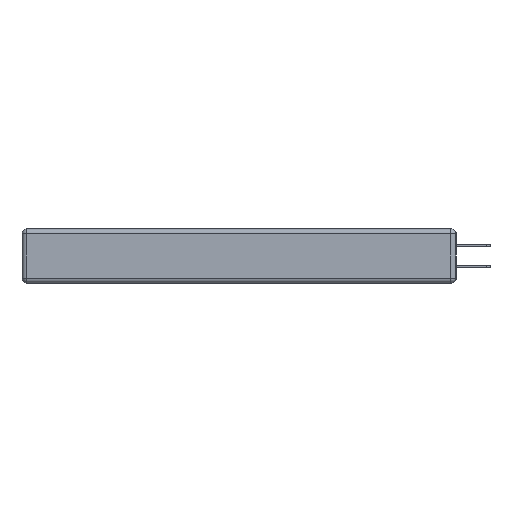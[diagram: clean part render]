
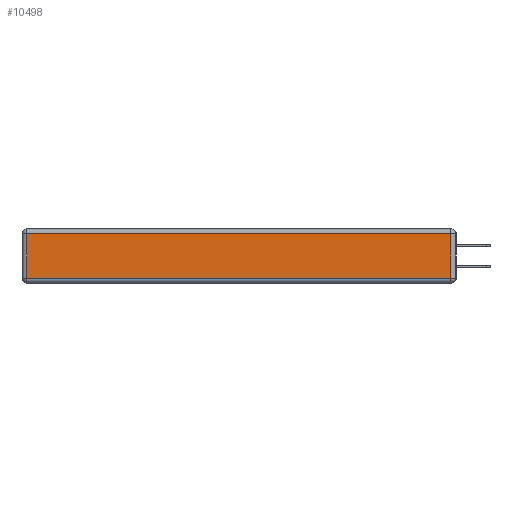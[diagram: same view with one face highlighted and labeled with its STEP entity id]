
A CAD part, left-side view. The second image highlights one B-rep face of the part: STEP entity #10498.
In plain terms, the highlighted planar face has unit normal (-1, 0, 0).
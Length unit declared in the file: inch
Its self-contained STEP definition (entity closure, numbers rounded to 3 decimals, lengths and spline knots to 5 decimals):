
#58 = CARTESIAN_POINT ( 'NONE',  ( 0., 0., -0.313 ) ) ;
#170 = CARTESIAN_POINT ( 'NONE',  ( 0., 0.03, -0.313 ) ) ;
#634 = ORIENTED_EDGE ( 'NONE', *, *, #1291, .T. ) ;
#694 = VECTOR ( 'NONE', #5084, 39.37008 ) ;
#899 = EDGE_CURVE ( 'NONE', #4016, #5563, #7367, .T. ) ;
#963 = VERTEX_POINT ( 'NONE', #13430 ) ;
#1291 = EDGE_CURVE ( 'NONE', #5563, #10634, #12744, .T. ) ;
#1335 = DIRECTION ( 'NONE',  ( 0., 0., 1. ) ) ;
#1717 = EDGE_LOOP ( 'NONE', ( #12720, #4150, #634, #4134 ) ) ;
#2519 = DIRECTION ( 'NONE',  ( -1., 0., 0. ) ) ;
#2928 = LINE ( 'NONE', #58, #13355 ) ;
#2948 = EDGE_CURVE ( 'NONE', #963, #4016, #2928, .T. ) ;
#3282 = DIRECTION ( 'NONE',  ( 0., -1., 0. ) ) ;
#3499 = CARTESIAN_POINT ( 'NONE',  ( 0., 2.75, -0.03 ) ) ;
#4013 = LINE ( 'NONE', #4587, #4160 ) ;
#4016 = VERTEX_POINT ( 'NONE', #170 ) ;
#4134 = ORIENTED_EDGE ( 'NONE', *, *, #13075, .T. ) ;
#4150 = ORIENTED_EDGE ( 'NONE', *, *, #899, .T. ) ;
#4160 = VECTOR ( 'NONE', #12890, 39.37008 ) ;
#4257 = AXIS2_PLACEMENT_3D ( 'NONE', #8532, #2519, #1335 ) ;
#4587 = CARTESIAN_POINT ( 'NONE',  ( 0., 2.72, -0.343 ) ) ;
#5084 = DIRECTION ( 'NONE',  ( 0., 0., 1. ) ) ;
#5414 = VECTOR ( 'NONE', #11889, 39.37008 ) ;
#5563 = VERTEX_POINT ( 'NONE', #9408 ) ;
#6183 = CARTESIAN_POINT ( 'NONE',  ( 0., 2.72, -0.03 ) ) ;
#7300 = CARTESIAN_POINT ( 'NONE',  ( 0., 0.03, -0.343 ) ) ;
#7367 = LINE ( 'NONE', #7300, #694 ) ;
#8532 = CARTESIAN_POINT ( 'NONE',  ( 0., 0., -0.343 ) ) ;
#9408 = CARTESIAN_POINT ( 'NONE',  ( 0., 0.03, -0.03 ) ) ;
#10498 = ADVANCED_FACE ( 'NONE', ( #11075 ), #11639, .T. ) ;
#10634 = VERTEX_POINT ( 'NONE', #6183 ) ;
#11075 = FACE_OUTER_BOUND ( 'NONE', #1717, .T. ) ;
#11639 = PLANE ( 'NONE',  #4257 ) ;
#11889 = DIRECTION ( 'NONE',  ( 0., 1., 0. ) ) ;
#12720 = ORIENTED_EDGE ( 'NONE', *, *, #2948, .T. ) ;
#12744 = LINE ( 'NONE', #3499, #5414 ) ;
#12890 = DIRECTION ( 'NONE',  ( 0., 0., -1. ) ) ;
#13075 = EDGE_CURVE ( 'NONE', #10634, #963, #4013, .T. ) ;
#13355 = VECTOR ( 'NONE', #3282, 39.37008 ) ;
#13430 = CARTESIAN_POINT ( 'NONE',  ( 0., 2.72, -0.313 ) ) ;
